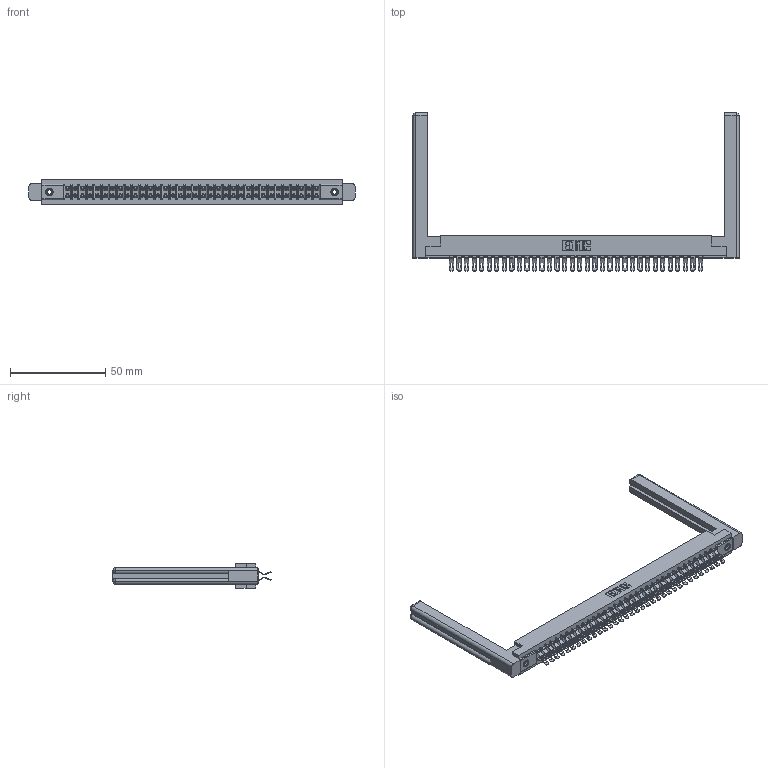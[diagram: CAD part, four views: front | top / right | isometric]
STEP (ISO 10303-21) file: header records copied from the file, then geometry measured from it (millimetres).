
FILE_DESCRIPTION (( 'STEP AP203' ), '1' );
FILE_NAME ('307-068-455-258.STEP', '2020-09-30T21:33:08', ( '' ), ( '' ), 'SwSTEP 2.0', 'SolidWorks 2020', '' );
FILE_SCHEMA (( 'CONFIG_CONTROL_DESIGN' ));
Length unit declared in the file: inch
Products named in the file (5): 345-250-001_345-250-001-102; 307-068-455-258; 307-220-058; 307 Part_.156 Dia Mounting Holes; 307-290-001_555
Assembly tree (73 placements, depth 2):
  307-068-455-258
    307 Part_.156 Dia Mounting Holes
    307-290-001_555  x68
    307-220-058  x2
    345-250-001_345-250-001-102  x2
Bounding box: 171.35 x 83.06 x 12.7 mm (x, y, z)
Volume: 25496.2 mm3; surface area: 28329.3 mm2
Topology: 73 solids, 73 shells, 4443 faces, 12985 edges, 8458 vertices
Faces by surface type: plane 2466, cylinder 1883, sphere 70, torus 12, cone 12
Entity records: 34392 total; most frequent: CARTESIAN_POINT 5653, ORIENTED_EDGE 5546, DIRECTION 5505, EDGE_CURVE 2773, VECTOR 2109, LINE 2109, VERTEX_POINT 1792, AXIS2_PLACEMENT_3D 1698
